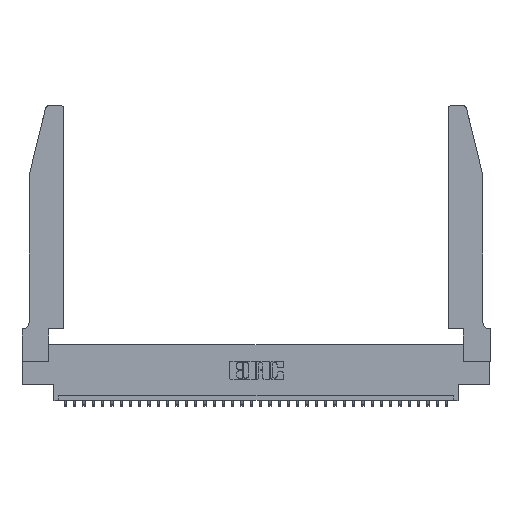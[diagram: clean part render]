
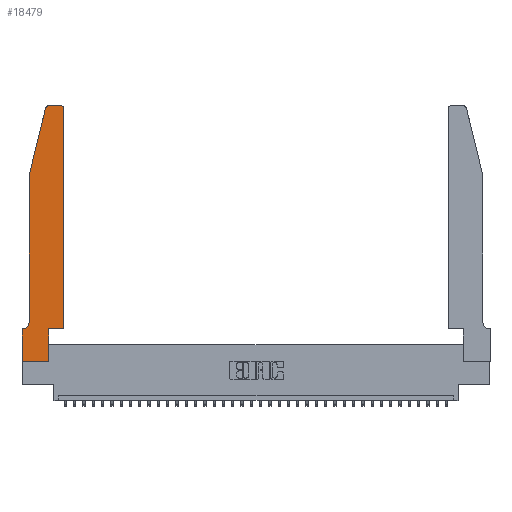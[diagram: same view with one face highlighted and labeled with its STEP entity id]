
A CAD part, top view. The second image highlights one B-rep face of the part: STEP entity #18479.
In plain terms, the highlighted planar face has unit normal (0, 0, 1).
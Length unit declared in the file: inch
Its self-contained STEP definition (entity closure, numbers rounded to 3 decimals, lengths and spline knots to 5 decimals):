
#39 = CARTESIAN_POINT ( 'NONE',  ( 0., 0., 0.37 ) ) ;
#50 = CIRCLE ( 'NONE', #7266, 0.03 ) ;
#694 = AXIS2_PLACEMENT_3D ( 'NONE', #18002, #26516, #9586 ) ;
#902 = VERTEX_POINT ( 'NONE', #25151 ) ;
#2519 = DIRECTION ( 'NONE',  ( -0.239, -0.971, 0. ) ) ;
#3268 = EDGE_CURVE ( 'NONE', #21786, #902, #20441, .T. ) ;
#3582 = LINE ( 'NONE', #28852, #35387 ) ;
#3606 = ORIENTED_EDGE ( 'NONE', *, *, #13177, .T. ) ;
#4843 = CARTESIAN_POINT ( 'NONE',  ( 0.0755, 0.35, 0.37 ) ) ;
#5146 = CIRCLE ( 'NONE', #694, 0.03 ) ;
#5930 = ORIENTED_EDGE ( 'NONE', *, *, #14102, .T. ) ;
#5959 = ORIENTED_EDGE ( 'NONE', *, *, #13059, .T. ) ;
#6293 = VERTEX_POINT ( 'NONE', #25274 ) ;
#6410 = DIRECTION ( 'NONE',  ( 0., -1., 0. ) ) ;
#6669 = LINE ( 'NONE', #25903, #26093 ) ;
#6931 = CARTESIAN_POINT ( 'NONE',  ( 0.2865, 0.35, 0.37 ) ) ;
#7015 = ORIENTED_EDGE ( 'NONE', *, *, #13512, .T. ) ;
#7144 = CARTESIAN_POINT ( 'NONE',  ( 0.0755, 0.42, 0.37 ) ) ;
#7266 = AXIS2_PLACEMENT_3D ( 'NONE', #21178, #13022, #13150 ) ;
#7802 = CARTESIAN_POINT ( 'NONE',  ( 0.0755, 2., 0.37 ) ) ;
#7892 = DIRECTION ( 'NONE',  ( 0., 0., 1. ) ) ;
#8126 = DIRECTION ( 'NONE',  ( 0., 0., -1. ) ) ;
#9537 = VERTEX_POINT ( 'NONE', #19504 ) ;
#9586 = DIRECTION ( 'NONE',  ( 1., 0., 0. ) ) ;
#9913 = ORIENTED_EDGE ( 'NONE', *, *, #13688, .T. ) ;
#10397 = CARTESIAN_POINT ( 'NONE',  ( 0., 0., 0.37 ) ) ;
#10472 = CARTESIAN_POINT ( 'NONE',  ( 0., 0.35, 0.37 ) ) ;
#11065 = EDGE_CURVE ( 'NONE', #30911, #20059, #17359, .T. ) ;
#11142 = FACE_OUTER_BOUND ( 'NONE', #29124, .T. ) ;
#11256 = CARTESIAN_POINT ( 'NONE',  ( 0.4505, 0.35, 0.37 ) ) ;
#11519 = AXIS2_PLACEMENT_3D ( 'NONE', #22214, #8126, #36456 ) ;
#11739 = ORIENTED_EDGE ( 'NONE', *, *, #25881, .T. ) ;
#11809 = AXIS2_PLACEMENT_3D ( 'NONE', #24796, #7892, #30269 ) ;
#12812 = LINE ( 'NONE', #28804, #33213 ) ;
#13022 = DIRECTION ( 'NONE',  ( 0., 0., 1. ) ) ;
#13059 = EDGE_CURVE ( 'NONE', #34239, #33515, #34526, .T. ) ;
#13150 = DIRECTION ( 'NONE',  ( 1., 0., 0. ) ) ;
#13177 = EDGE_CURVE ( 'NONE', #6293, #33713, #6669, .T. ) ;
#13227 = DIRECTION ( 'NONE',  ( 1., 0., 0. ) ) ;
#13512 = EDGE_CURVE ( 'NONE', #9537, #19963, #3582, .T. ) ;
#13637 = VECTOR ( 'NONE', #13227, 39.37008 ) ;
#13688 = EDGE_CURVE ( 'NONE', #35449, #9537, #50, .T. ) ;
#14102 = EDGE_CURVE ( 'NONE', #33713, #18555, #17193, .T. ) ;
#14265 = LINE ( 'NONE', #4843, #29773 ) ;
#15436 = EDGE_CURVE ( 'NONE', #902, #6293, #22900, .T. ) ;
#15638 = ORIENTED_EDGE ( 'NONE', *, *, #18466, .T. ) ;
#17193 = LINE ( 'NONE', #11256, #20265 ) ;
#17359 = CIRCLE ( 'NONE', #11519, 0.07 ) ;
#17380 = DIRECTION ( 'NONE',  ( 0., 1., 0. ) ) ;
#18002 = CARTESIAN_POINT ( 'NONE',  ( 0.284, 2.72, 0.37 ) ) ;
#18466 = EDGE_CURVE ( 'NONE', #20059, #21786, #14265, .T. ) ;
#18479 = ADVANCED_FACE ( 'NONE', ( #11142 ), #33247, .T. ) ;
#18555 = VERTEX_POINT ( 'NONE', #24674 ) ;
#19504 = CARTESIAN_POINT ( 'NONE',  ( 0.4205, 2.75, 0.37 ) ) ;
#19963 = VERTEX_POINT ( 'NONE', #24339 ) ;
#20059 = VERTEX_POINT ( 'NONE', #24853 ) ;
#20265 = VECTOR ( 'NONE', #28714, 39.37008 ) ;
#20441 = LINE ( 'NONE', #39, #21773 ) ;
#20510 = VECTOR ( 'NONE', #6410, 39.37008 ) ;
#21178 = CARTESIAN_POINT ( 'NONE',  ( 0.4205, 2.72, 0.37 ) ) ;
#21356 = ORIENTED_EDGE ( 'NONE', *, *, #11065, .T. ) ;
#21596 = DIRECTION ( 'NONE',  ( -1., 0., 0. ) ) ;
#21773 = VECTOR ( 'NONE', #33476, 39.37008 ) ;
#21786 = VERTEX_POINT ( 'NONE', #10472 ) ;
#22214 = CARTESIAN_POINT ( 'NONE',  ( 0.0055, 0.42, 0.37 ) ) ;
#22900 = LINE ( 'NONE', #10397, #13637 ) ;
#24339 = CARTESIAN_POINT ( 'NONE',  ( 0.284, 2.75, 0.37 ) ) ;
#24674 = CARTESIAN_POINT ( 'NONE',  ( 0.4505, 0.35, 0.37 ) ) ;
#24796 = CARTESIAN_POINT ( 'NONE',  ( 0., 0.35, 0.37 ) ) ;
#24853 = CARTESIAN_POINT ( 'NONE',  ( 0.0055, 0.35, 0.37 ) ) ;
#25151 = CARTESIAN_POINT ( 'NONE',  ( 0., 0., 0.37 ) ) ;
#25274 = CARTESIAN_POINT ( 'NONE',  ( 0.2865, 0., 0.37 ) ) ;
#25796 = LINE ( 'NONE', #34595, #20510 ) ;
#25881 = EDGE_CURVE ( 'NONE', #19963, #34239, #5146, .T. ) ;
#25903 = CARTESIAN_POINT ( 'NONE',  ( 0.2865, 0.35, 0.37 ) ) ;
#25939 = CARTESIAN_POINT ( 'NONE',  ( 0.0755, 2., 0.37 ) ) ;
#26053 = DIRECTION ( 'NONE',  ( 0., 1., 0. ) ) ;
#26093 = VECTOR ( 'NONE', #17380, 39.37008 ) ;
#26363 = DIRECTION ( 'NONE',  ( -1., 0., 0. ) ) ;
#26516 = DIRECTION ( 'NONE',  ( 0., 0., 1. ) ) ;
#26827 = CARTESIAN_POINT ( 'NONE',  ( 0.4505, 2.72, 0.37 ) ) ;
#27450 = VECTOR ( 'NONE', #2519, 39.37008 ) ;
#28323 = ORIENTED_EDGE ( 'NONE', *, *, #28425, .T. ) ;
#28425 = EDGE_CURVE ( 'NONE', #18555, #35449, #12812, .T. ) ;
#28714 = DIRECTION ( 'NONE',  ( 1., 0., 0. ) ) ;
#28804 = CARTESIAN_POINT ( 'NONE',  ( 0.4505, 0.35, 0.37 ) ) ;
#28852 = CARTESIAN_POINT ( 'NONE',  ( 0.2605, 2.75, 0.37 ) ) ;
#29124 = EDGE_LOOP ( 'NONE', ( #7015, #11739, #5959, #32322, #21356, #15638, #34961, #31827, #3606, #5930, #28323, #9913 ) ) ;
#29773 = VECTOR ( 'NONE', #21596, 39.37008 ) ;
#30269 = DIRECTION ( 'NONE',  ( 1., 0., 0. ) ) ;
#30911 = VERTEX_POINT ( 'NONE', #7144 ) ;
#31827 = ORIENTED_EDGE ( 'NONE', *, *, #15436, .T. ) ;
#32233 = CARTESIAN_POINT ( 'NONE',  ( 0.25487, 2.72718, 0.37 ) ) ;
#32322 = ORIENTED_EDGE ( 'NONE', *, *, #35893, .T. ) ;
#33213 = VECTOR ( 'NONE', #26053, 39.37008 ) ;
#33247 = PLANE ( 'NONE',  #11809 ) ;
#33476 = DIRECTION ( 'NONE',  ( 0., -1., 0. ) ) ;
#33515 = VERTEX_POINT ( 'NONE', #25939 ) ;
#33713 = VERTEX_POINT ( 'NONE', #6931 ) ;
#34239 = VERTEX_POINT ( 'NONE', #32233 ) ;
#34526 = LINE ( 'NONE', #7802, #27450 ) ;
#34595 = CARTESIAN_POINT ( 'NONE',  ( 0.0755, 2., 0.37 ) ) ;
#34961 = ORIENTED_EDGE ( 'NONE', *, *, #3268, .T. ) ;
#35387 = VECTOR ( 'NONE', #26363, 39.37008 ) ;
#35449 = VERTEX_POINT ( 'NONE', #26827 ) ;
#35893 = EDGE_CURVE ( 'NONE', #33515, #30911, #25796, .T. ) ;
#36456 = DIRECTION ( 'NONE',  ( -1., 0., 0. ) ) ;
